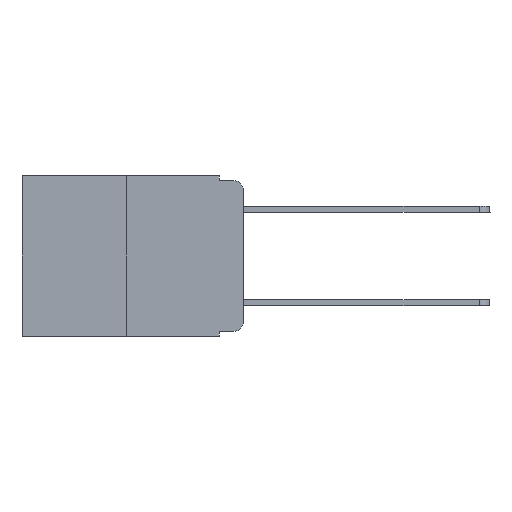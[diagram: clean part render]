
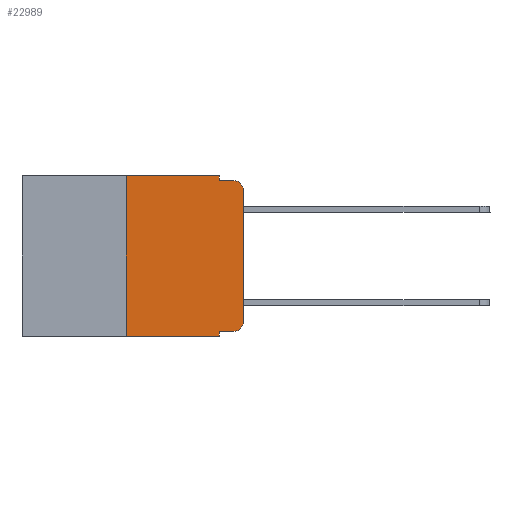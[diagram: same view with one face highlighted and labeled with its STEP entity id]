
A CAD part, left-side view. The second image highlights one B-rep face of the part: STEP entity #22989.
In plain terms, the highlighted planar face has unit normal (-1, 0, 0).
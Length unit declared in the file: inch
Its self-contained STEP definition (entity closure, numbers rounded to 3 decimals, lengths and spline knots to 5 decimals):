
#368 = EDGE_CURVE ( 'NONE', #3961, #5573, #13424, .T. ) ;
#434 = DIRECTION ( 'NONE',  ( 0., 0., -1. ) ) ;
#663 = CARTESIAN_POINT ( 'NONE',  ( 0., 0.02, -0.03 ) ) ;
#991 = AXIS2_PLACEMENT_3D ( 'NONE', #14769, #19233, #434 ) ;
#2007 = CARTESIAN_POINT ( 'NONE',  ( 0., 0.25, -0.343 ) ) ;
#3031 = CARTESIAN_POINT ( 'NONE',  ( 0., 0., -0.313 ) ) ;
#3051 = ORIENTED_EDGE ( 'NONE', *, *, #18567, .T. ) ;
#3116 = VERTEX_POINT ( 'NONE', #18267 ) ;
#3140 = FACE_OUTER_BOUND ( 'NONE', #6590, .T. ) ;
#3961 = VERTEX_POINT ( 'NONE', #15985 ) ;
#4397 = CARTESIAN_POINT ( 'NONE',  ( 0., 0., -0.03 ) ) ;
#4449 = VERTEX_POINT ( 'NONE', #17769 ) ;
#5037 = LINE ( 'NONE', #16825, #23807 ) ;
#5193 = VECTOR ( 'NONE', #22896, 39.37008 ) ;
#5573 = VERTEX_POINT ( 'NONE', #13306 ) ;
#5700 = ORIENTED_EDGE ( 'NONE', *, *, #21423, .T. ) ;
#5997 = LINE ( 'NONE', #23516, #23062 ) ;
#6258 = CARTESIAN_POINT ( 'NONE',  ( 0., 0.051, -0.333 ) ) ;
#6590 = EDGE_LOOP ( 'NONE', ( #16032, #19652, #7374, #16508, #22933, #22408, #5700, #13710, #3051, #10978 ) ) ;
#7060 = PLANE ( 'NONE',  #991 ) ;
#7097 = CARTESIAN_POINT ( 'NONE',  ( 0., 0.02, -0.313 ) ) ;
#7346 = VECTOR ( 'NONE', #9396, 39.37008 ) ;
#7374 = ORIENTED_EDGE ( 'NONE', *, *, #8197, .F. ) ;
#7935 = CARTESIAN_POINT ( 'NONE',  ( 0., 0.02, -0.333 ) ) ;
#7982 = VERTEX_POINT ( 'NONE', #7935 ) ;
#7990 = AXIS2_PLACEMENT_3D ( 'NONE', #7097, #21146, #11006 ) ;
#8197 = EDGE_CURVE ( 'NONE', #22791, #3116, #5037, .T. ) ;
#8383 = DIRECTION ( 'NONE',  ( 0., 0., -1. ) ) ;
#8510 = DIRECTION ( 'NONE',  ( -1., 0., 0. ) ) ;
#9256 = AXIS2_PLACEMENT_3D ( 'NONE', #663, #8510, #8383 ) ;
#9396 = DIRECTION ( 'NONE',  ( 0., 0., -1. ) ) ;
#9693 = EDGE_CURVE ( 'NONE', #15823, #21510, #15117, .T. ) ;
#10118 = CARTESIAN_POINT ( 'NONE',  ( 0., 0.051, 0. ) ) ;
#10324 = CARTESIAN_POINT ( 'NONE',  ( 0., 0.051, -0.01 ) ) ;
#10978 = ORIENTED_EDGE ( 'NONE', *, *, #12785, .T. ) ;
#11006 = DIRECTION ( 'NONE',  ( 0., 0., -1. ) ) ;
#11122 = EDGE_CURVE ( 'NONE', #15959, #4449, #5997, .T. ) ;
#11197 = EDGE_CURVE ( 'NONE', #4449, #15640, #12167, .T. ) ;
#11258 = EDGE_CURVE ( 'NONE', #21510, #3116, #22699, .T. ) ;
#11475 = CARTESIAN_POINT ( 'NONE',  ( 0., 0.473, -0.343 ) ) ;
#11919 = DIRECTION ( 'NONE',  ( 0., -1., 0. ) ) ;
#12167 = LINE ( 'NONE', #19946, #12896 ) ;
#12785 = EDGE_CURVE ( 'NONE', #7982, #15823, #20573, .T. ) ;
#12896 = VECTOR ( 'NONE', #11919, 39.37008 ) ;
#13306 = CARTESIAN_POINT ( 'NONE',  ( 0., 0.051, -0.343 ) ) ;
#13361 = LINE ( 'NONE', #11475, #18775 ) ;
#13424 = LINE ( 'NONE', #18947, #7346 ) ;
#13456 = LINE ( 'NONE', #6258, #22802 ) ;
#13649 = DIRECTION ( 'NONE',  ( 0., 0., -1. ) ) ;
#13710 = ORIENTED_EDGE ( 'NONE', *, *, #368, .F. ) ;
#14269 = CARTESIAN_POINT ( 'NONE',  ( 0., 0.051, 0. ) ) ;
#14769 = CARTESIAN_POINT ( 'NONE',  ( 0., 0.473, 0. ) ) ;
#14866 = CARTESIAN_POINT ( 'NONE',  ( 0., 0., 0. ) ) ;
#15117 = LINE ( 'NONE', #14866, #5193 ) ;
#15640 = VERTEX_POINT ( 'NONE', #14269 ) ;
#15823 = VERTEX_POINT ( 'NONE', #3031 ) ;
#15959 = VERTEX_POINT ( 'NONE', #2007 ) ;
#15985 = CARTESIAN_POINT ( 'NONE',  ( 0., 0.051, -0.333 ) ) ;
#16032 = ORIENTED_EDGE ( 'NONE', *, *, #9693, .T. ) ;
#16508 = ORIENTED_EDGE ( 'NONE', *, *, #20661, .F. ) ;
#16825 = CARTESIAN_POINT ( 'NONE',  ( 0., 0.051, -0.01 ) ) ;
#17769 = CARTESIAN_POINT ( 'NONE',  ( 0., 0.25, 0. ) ) ;
#18267 = CARTESIAN_POINT ( 'NONE',  ( 0., 0.02, -0.01 ) ) ;
#18567 = EDGE_CURVE ( 'NONE', #3961, #7982, #13456, .T. ) ;
#18775 = VECTOR ( 'NONE', #19492, 39.37008 ) ;
#18947 = CARTESIAN_POINT ( 'NONE',  ( 0., 0.051, 0. ) ) ;
#19233 = DIRECTION ( 'NONE',  ( 1., 0., 0. ) ) ;
#19422 = LINE ( 'NONE', #10118, #20788 ) ;
#19492 = DIRECTION ( 'NONE',  ( 0., -1., 0. ) ) ;
#19589 = DIRECTION ( 'NONE',  ( 0., -1., 0. ) ) ;
#19652 = ORIENTED_EDGE ( 'NONE', *, *, #11258, .T. ) ;
#19946 = CARTESIAN_POINT ( 'NONE',  ( 0., 0.473, 0. ) ) ;
#20573 = CIRCLE ( 'NONE', #7990, 0.02 ) ;
#20661 = EDGE_CURVE ( 'NONE', #15640, #22791, #19422, .T. ) ;
#20788 = VECTOR ( 'NONE', #13649, 39.37008 ) ;
#21146 = DIRECTION ( 'NONE',  ( -1., 0., 0. ) ) ;
#21354 = DIRECTION ( 'NONE',  ( 0., 0., 1. ) ) ;
#21423 = EDGE_CURVE ( 'NONE', #15959, #5573, #13361, .T. ) ;
#21510 = VERTEX_POINT ( 'NONE', #4397 ) ;
#22408 = ORIENTED_EDGE ( 'NONE', *, *, #11122, .F. ) ;
#22699 = CIRCLE ( 'NONE', #9256, 0.02 ) ;
#22791 = VERTEX_POINT ( 'NONE', #10324 ) ;
#22802 = VECTOR ( 'NONE', #19589, 39.37008 ) ;
#22896 = DIRECTION ( 'NONE',  ( 0., 0., 1. ) ) ;
#22933 = ORIENTED_EDGE ( 'NONE', *, *, #11197, .F. ) ;
#22989 = ADVANCED_FACE ( 'NONE', ( #3140 ), #7060, .F. ) ;
#23062 = VECTOR ( 'NONE', #21354, 39.37008 ) ;
#23516 = CARTESIAN_POINT ( 'NONE',  ( 0., 0.25, 0. ) ) ;
#23807 = VECTOR ( 'NONE', #24574, 39.37008 ) ;
#24574 = DIRECTION ( 'NONE',  ( 0., -1., 0. ) ) ;
